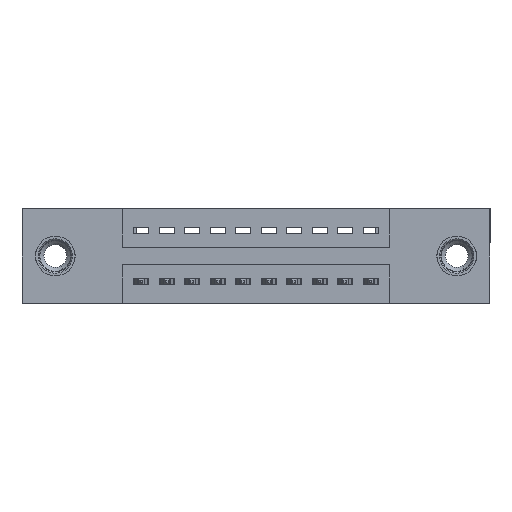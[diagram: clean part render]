
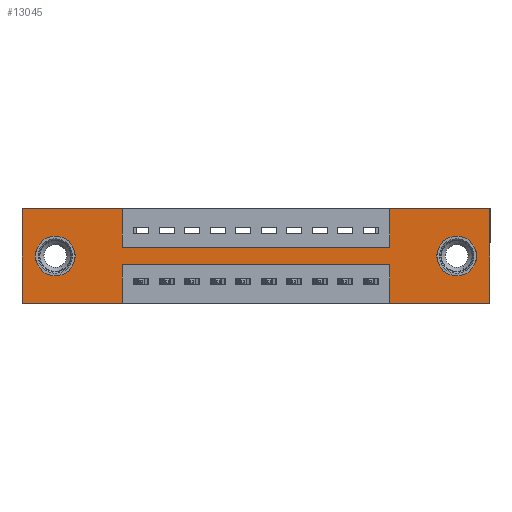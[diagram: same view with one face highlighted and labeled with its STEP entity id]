
A CAD part, front view. The second image highlights one B-rep face of the part: STEP entity #13045.
In plain terms, the highlighted planar face has unit normal (0, -1, 0).
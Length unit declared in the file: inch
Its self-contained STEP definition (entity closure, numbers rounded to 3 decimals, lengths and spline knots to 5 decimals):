
#20 = VERTEX_POINT ( 'NONE', #9822 ) ;
#110 = VERTEX_POINT ( 'NONE', #6480 ) ;
#123 = CARTESIAN_POINT ( 'NONE',  ( 1.4425, 0., -0.37 ) ) ;
#186 = CARTESIAN_POINT ( 'NONE',  ( 0., 0., -0.37 ) ) ;
#187 = EDGE_LOOP ( 'NONE', ( #8193, #5641 ) ) ;
#257 = CARTESIAN_POINT ( 'NONE',  ( 0.3925, 0., -0.37 ) ) ;
#436 = DIRECTION ( 'NONE',  ( 0., 0., 1. ) ) ;
#514 = CARTESIAN_POINT ( 'NONE',  ( 0., 0., -0.37 ) ) ;
#651 = VECTOR ( 'NONE', #12198, 39.37008 ) ;
#683 = ORIENTED_EDGE ( 'NONE', *, *, #7906, .F. ) ;
#824 = AXIS2_PLACEMENT_3D ( 'NONE', #514, #6870, #7962 ) ;
#916 = DIRECTION ( 'NONE',  ( 0., 1., 0. ) ) ;
#1438 = FACE_BOUND ( 'NONE', #187, .T. ) ;
#1578 = CIRCLE ( 'NONE', #9141, 0.078 ) ;
#1580 = VERTEX_POINT ( 'NONE', #5891 ) ;
#1642 = CIRCLE ( 'NONE', #2468, 0.078 ) ;
#1977 = VERTEX_POINT ( 'NONE', #3295 ) ;
#2021 = CARTESIAN_POINT ( 'NONE',  ( 1.4425, 0., -0.22 ) ) ;
#2026 = DIRECTION ( 'NONE',  ( 0., 0., -1. ) ) ;
#2031 = CARTESIAN_POINT ( 'NONE',  ( 0.3925, 0., -0.37 ) ) ;
#2079 = LINE ( 'NONE', #8997, #11730 ) ;
#2465 = EDGE_CURVE ( 'NONE', #5237, #8753, #3454, .T. ) ;
#2468 = AXIS2_PLACEMENT_3D ( 'NONE', #11866, #916, #2026 ) ;
#2543 = VECTOR ( 'NONE', #12609, 39.37008 ) ;
#2567 = EDGE_CURVE ( 'NONE', #8065, #8603, #10406, .T. ) ;
#2764 = EDGE_LOOP ( 'NONE', ( #10984, #13246 ) ) ;
#2824 = CARTESIAN_POINT ( 'NONE',  ( 0.3925, 0., 0. ) ) ;
#2919 = EDGE_CURVE ( 'NONE', #110, #20, #10905, .T. ) ;
#3190 = EDGE_CURVE ( 'NONE', #10177, #5983, #13267, .T. ) ;
#3295 = CARTESIAN_POINT ( 'NONE',  ( 0.13, 0., -0.263 ) ) ;
#3431 = ORIENTED_EDGE ( 'NONE', *, *, #11639, .F. ) ;
#3451 = DIRECTION ( 'NONE',  ( 0., 0., -1. ) ) ;
#3454 = LINE ( 'NONE', #2031, #13636 ) ;
#3659 = CARTESIAN_POINT ( 'NONE',  ( 1.835, 0., -0.37 ) ) ;
#3703 = EDGE_CURVE ( 'NONE', #1580, #1977, #1578, .T. ) ;
#3798 = CARTESIAN_POINT ( 'NONE',  ( 0., 0., -0.37 ) ) ;
#3883 = CARTESIAN_POINT ( 'NONE',  ( 0., 0., 0. ) ) ;
#3957 = EDGE_CURVE ( 'NONE', #1977, #1580, #8158, .T. ) ;
#4004 = EDGE_CURVE ( 'NONE', #5121, #8065, #2079, .T. ) ;
#4096 = CARTESIAN_POINT ( 'NONE',  ( 1.835, 0., 0. ) ) ;
#4309 = FACE_BOUND ( 'NONE', #2764, .T. ) ;
#4325 = DIRECTION ( 'NONE',  ( 0., 0., -1. ) ) ;
#4530 = CARTESIAN_POINT ( 'NONE',  ( 1.4425, 0., -0.37 ) ) ;
#4564 = CARTESIAN_POINT ( 'NONE',  ( 0., 0., 0. ) ) ;
#4648 = VECTOR ( 'NONE', #8777, 39.37008 ) ;
#4921 = DIRECTION ( 'NONE',  ( 1., 0., 0. ) ) ;
#4974 = EDGE_CURVE ( 'NONE', #9331, #11334, #11182, .T. ) ;
#4990 = DIRECTION ( 'NONE',  ( -1., 0., 0. ) ) ;
#5068 = CARTESIAN_POINT ( 'NONE',  ( 1.835, 0., 0. ) ) ;
#5121 = VERTEX_POINT ( 'NONE', #7504 ) ;
#5237 = VERTEX_POINT ( 'NONE', #12115 ) ;
#5300 = ORIENTED_EDGE ( 'NONE', *, *, #7921, .F. ) ;
#5308 = CARTESIAN_POINT ( 'NONE',  ( 0.3925, 0., -0.22 ) ) ;
#5527 = ORIENTED_EDGE ( 'NONE', *, *, #2567, .F. ) ;
#5641 = ORIENTED_EDGE ( 'NONE', *, *, #3957, .T. ) ;
#5841 = VECTOR ( 'NONE', #4990, 39.37008 ) ;
#5891 = CARTESIAN_POINT ( 'NONE',  ( 0.13, 0., -0.107 ) ) ;
#5972 = ORIENTED_EDGE ( 'NONE', *, *, #4004, .F. ) ;
#5983 = VERTEX_POINT ( 'NONE', #10620 ) ;
#6341 = DIRECTION ( 'NONE',  ( 0., 0., 1. ) ) ;
#6480 = CARTESIAN_POINT ( 'NONE',  ( 1.4425, 0., -0.15 ) ) ;
#6533 = ORIENTED_EDGE ( 'NONE', *, *, #2919, .F. ) ;
#6564 = CARTESIAN_POINT ( 'NONE',  ( 1.705, 0., -0.107 ) ) ;
#6697 = ORIENTED_EDGE ( 'NONE', *, *, #12938, .F. ) ;
#6863 = EDGE_CURVE ( 'NONE', #11334, #7936, #7703, .T. ) ;
#6870 = DIRECTION ( 'NONE',  ( 0., -1., 0. ) ) ;
#7054 = DIRECTION ( 'NONE',  ( 0., 0., 1. ) ) ;
#7106 = EDGE_CURVE ( 'NONE', #8753, #5121, #13665, .T. ) ;
#7504 = CARTESIAN_POINT ( 'NONE',  ( 0., 0., -0.37 ) ) ;
#7679 = VECTOR ( 'NONE', #6341, 39.37008 ) ;
#7697 = LINE ( 'NONE', #4530, #10258 ) ;
#7703 = LINE ( 'NONE', #186, #13305 ) ;
#7745 = DIRECTION ( 'NONE',  ( -1., 0., 0. ) ) ;
#7804 = DIRECTION ( 'NONE',  ( 0., 1., 0. ) ) ;
#7810 = VERTEX_POINT ( 'NONE', #10121 ) ;
#7906 = EDGE_CURVE ( 'NONE', #11208, #5237, #13102, .T. ) ;
#7921 = EDGE_CURVE ( 'NONE', #7810, #110, #9750, .T. ) ;
#7936 = VERTEX_POINT ( 'NONE', #123 ) ;
#7962 = DIRECTION ( 'NONE',  ( 0., 0., -1. ) ) ;
#8062 = CARTESIAN_POINT ( 'NONE',  ( 0., 0., 0. ) ) ;
#8065 = VERTEX_POINT ( 'NONE', #3883 ) ;
#8158 = CIRCLE ( 'NONE', #12949, 0.078 ) ;
#8193 = ORIENTED_EDGE ( 'NONE', *, *, #3703, .T. ) ;
#8522 = CARTESIAN_POINT ( 'NONE',  ( 0.3925, 0., 0. ) ) ;
#8592 = LINE ( 'NONE', #8522, #651 ) ;
#8603 = VERTEX_POINT ( 'NONE', #2824 ) ;
#8731 = DIRECTION ( 'NONE',  ( -1., 0., 0. ) ) ;
#8736 = ORIENTED_EDGE ( 'NONE', *, *, #7106, .F. ) ;
#8753 = VERTEX_POINT ( 'NONE', #257 ) ;
#8777 = DIRECTION ( 'NONE',  ( 1., 0., 0. ) ) ;
#8914 = CARTESIAN_POINT ( 'NONE',  ( 1.705, 0., -0.185 ) ) ;
#8997 = CARTESIAN_POINT ( 'NONE',  ( 0., 0., 0. ) ) ;
#9141 = AXIS2_PLACEMENT_3D ( 'NONE', #13357, #13560, #7054 ) ;
#9331 = VERTEX_POINT ( 'NONE', #4096 ) ;
#9474 = LINE ( 'NONE', #8062, #9954 ) ;
#9723 = ORIENTED_EDGE ( 'NONE', *, *, #6863, .F. ) ;
#9734 = VECTOR ( 'NONE', #13128, 39.37008 ) ;
#9750 = LINE ( 'NONE', #12205, #9734 ) ;
#9822 = CARTESIAN_POINT ( 'NONE',  ( 1.4425, 0., 0. ) ) ;
#9954 = VECTOR ( 'NONE', #4921, 39.37008 ) ;
#10085 = DIRECTION ( 'NONE',  ( 0., 0., 1. ) ) ;
#10121 = CARTESIAN_POINT ( 'NONE',  ( 0.3925, 0., -0.15 ) ) ;
#10177 = VERTEX_POINT ( 'NONE', #6564 ) ;
#10258 = VECTOR ( 'NONE', #13137, 39.37008 ) ;
#10406 = LINE ( 'NONE', #4564, #4648 ) ;
#10620 = CARTESIAN_POINT ( 'NONE',  ( 1.705, 0., -0.263 ) ) ;
#10905 = LINE ( 'NONE', #13662, #7679 ) ;
#10984 = ORIENTED_EDGE ( 'NONE', *, *, #3190, .T. ) ;
#10999 = ORIENTED_EDGE ( 'NONE', *, *, #4974, .F. ) ;
#11064 = EDGE_CURVE ( 'NONE', #20, #9331, #9474, .T. ) ;
#11170 = DIRECTION ( 'NONE',  ( 0., 1., 0. ) ) ;
#11182 = LINE ( 'NONE', #5068, #2543 ) ;
#11208 = VERTEX_POINT ( 'NONE', #2021 ) ;
#11334 = VERTEX_POINT ( 'NONE', #3659 ) ;
#11615 = VECTOR ( 'NONE', #8731, 39.37008 ) ;
#11639 = EDGE_CURVE ( 'NONE', #8603, #7810, #8592, .T. ) ;
#11730 = VECTOR ( 'NONE', #10085, 39.37008 ) ;
#11837 = ORIENTED_EDGE ( 'NONE', *, *, #2465, .F. ) ;
#11866 = CARTESIAN_POINT ( 'NONE',  ( 1.705, 0., -0.185 ) ) ;
#12115 = CARTESIAN_POINT ( 'NONE',  ( 0.3925, 0., -0.22 ) ) ;
#12126 = FACE_OUTER_BOUND ( 'NONE', #13633, .T. ) ;
#12198 = DIRECTION ( 'NONE',  ( 0., 0., -1. ) ) ;
#12205 = CARTESIAN_POINT ( 'NONE',  ( 0.3925, 0., -0.15 ) ) ;
#12391 = ORIENTED_EDGE ( 'NONE', *, *, #11064, .F. ) ;
#12445 = EDGE_CURVE ( 'NONE', #5983, #10177, #1642, .T. ) ;
#12509 = AXIS2_PLACEMENT_3D ( 'NONE', #8914, #7804, #3451 ) ;
#12609 = DIRECTION ( 'NONE',  ( 0., 0., -1. ) ) ;
#12938 = EDGE_CURVE ( 'NONE', #7936, #11208, #7697, .T. ) ;
#12949 = AXIS2_PLACEMENT_3D ( 'NONE', #13390, #11170, #436 ) ;
#13045 = ADVANCED_FACE ( 'NONE', ( #4309, #1438, #12126 ), #13484, .T. ) ;
#13102 = LINE ( 'NONE', #5308, #11615 ) ;
#13128 = DIRECTION ( 'NONE',  ( 1., 0., 0. ) ) ;
#13137 = DIRECTION ( 'NONE',  ( 0., 0., 1. ) ) ;
#13246 = ORIENTED_EDGE ( 'NONE', *, *, #12445, .T. ) ;
#13267 = CIRCLE ( 'NONE', #12509, 0.078 ) ;
#13305 = VECTOR ( 'NONE', #7745, 39.37008 ) ;
#13357 = CARTESIAN_POINT ( 'NONE',  ( 0.13, 0., -0.185 ) ) ;
#13390 = CARTESIAN_POINT ( 'NONE',  ( 0.13, 0., -0.185 ) ) ;
#13484 = PLANE ( 'NONE',  #824 ) ;
#13560 = DIRECTION ( 'NONE',  ( 0., 1., 0. ) ) ;
#13633 = EDGE_LOOP ( 'NONE', ( #11837, #683, #6697, #9723, #10999, #12391, #6533, #5300, #3431, #5527, #5972, #8736 ) ) ;
#13636 = VECTOR ( 'NONE', #4325, 39.37008 ) ;
#13662 = CARTESIAN_POINT ( 'NONE',  ( 1.4425, 0., 0. ) ) ;
#13665 = LINE ( 'NONE', #3798, #5841 ) ;
